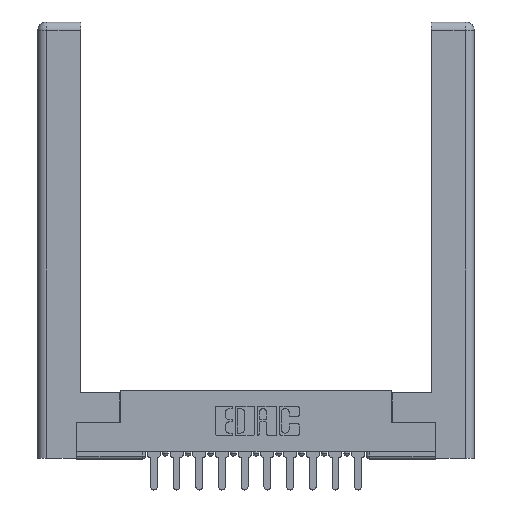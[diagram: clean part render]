
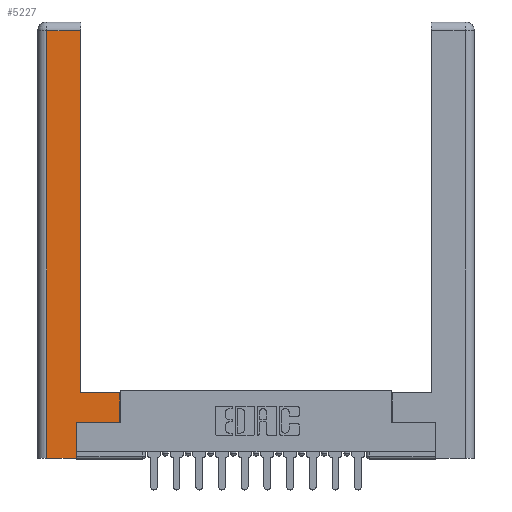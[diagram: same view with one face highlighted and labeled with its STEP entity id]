
A CAD part, top view. The second image highlights one B-rep face of the part: STEP entity #5227.
In plain terms, the highlighted planar face has unit normal (0, 0, 1).
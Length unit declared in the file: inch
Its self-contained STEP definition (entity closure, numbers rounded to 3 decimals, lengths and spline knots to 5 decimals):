
#291 = CARTESIAN_POINT ( 'NONE',  ( 0.0615, 0., 0. ) ) ;
#325 = CARTESIAN_POINT ( 'NONE',  ( 0.265, 0., 0. ) ) ;
#368 = ORIENTED_EDGE ( 'NONE', *, *, #6284, .T. ) ;
#783 = VERTEX_POINT ( 'NONE', #10600 ) ;
#956 = CARTESIAN_POINT ( 'NONE',  ( 0.565, 0.245, 0. ) ) ;
#1530 = VECTOR ( 'NONE', #2260, 39.37008 ) ;
#1540 = VECTOR ( 'NONE', #11471, 39.37008 ) ;
#1660 = ORIENTED_EDGE ( 'NONE', *, *, #10206, .T. ) ;
#2072 = ORIENTED_EDGE ( 'NONE', *, *, #11673, .T. ) ;
#2087 = LINE ( 'NONE', #2231, #9474 ) ;
#2155 = DIRECTION ( 'NONE',  ( -1., 0., 0. ) ) ;
#2202 = DIRECTION ( 'NONE',  ( -1., 0., 0. ) ) ;
#2231 = CARTESIAN_POINT ( 'NONE',  ( 0.295, 3., 0. ) ) ;
#2260 = DIRECTION ( 'NONE',  ( 0., 1., 0. ) ) ;
#2530 = EDGE_CURVE ( 'NONE', #13134, #783, #7236, .T. ) ;
#2780 = LINE ( 'NONE', #5709, #1530 ) ;
#2924 = EDGE_CURVE ( 'NONE', #9411, #13294, #2087, .T. ) ;
#3008 = EDGE_CURVE ( 'NONE', #9317, #10357, #3397, .T. ) ;
#3238 = DIRECTION ( 'NONE',  ( 0., 1., 0. ) ) ;
#3397 = LINE ( 'NONE', #10175, #13503 ) ;
#3718 = CARTESIAN_POINT ( 'NONE',  ( 0.565, 0.45, 0. ) ) ;
#3811 = DIRECTION ( 'NONE',  ( 1., 0., 0. ) ) ;
#3886 = DIRECTION ( 'NONE',  ( 0., 0., -1. ) ) ;
#4324 = DIRECTION ( 'NONE',  ( 0., 1., 0. ) ) ;
#4502 = EDGE_CURVE ( 'NONE', #8087, #12818, #2780, .T. ) ;
#4535 = VECTOR ( 'NONE', #2155, 39.37008 ) ;
#4922 = DIRECTION ( 'NONE',  ( 0., -1., 0. ) ) ;
#5039 = FACE_OUTER_BOUND ( 'NONE', #12690, .T. ) ;
#5227 = ADVANCED_FACE ( 'NONE', ( #5039 ), #9749, .F. ) ;
#5663 = CARTESIAN_POINT ( 'NONE',  ( 0.0615, 2.94, 0. ) ) ;
#5709 = CARTESIAN_POINT ( 'NONE',  ( 0.265, 0.245, 0. ) ) ;
#6284 = EDGE_CURVE ( 'NONE', #12818, #9317, #10082, .T. ) ;
#6409 = CARTESIAN_POINT ( 'NONE',  ( 0.0615, 2.94, 0. ) ) ;
#6525 = ORIENTED_EDGE ( 'NONE', *, *, #2924, .T. ) ;
#6530 = VECTOR ( 'NONE', #4922, 39.37008 ) ;
#6611 = CARTESIAN_POINT ( 'NONE',  ( 0.565, 0.245, 0. ) ) ;
#6668 = AXIS2_PLACEMENT_3D ( 'NONE', #14415, #3886, #8582 ) ;
#7236 = LINE ( 'NONE', #291, #6530 ) ;
#7510 = LINE ( 'NONE', #325, #11706 ) ;
#7615 = ORIENTED_EDGE ( 'NONE', *, *, #4502, .T. ) ;
#7645 = CARTESIAN_POINT ( 'NONE',  ( 0.295, 0.45, 0. ) ) ;
#7831 = CARTESIAN_POINT ( 'NONE',  ( 0.295, 0.45, 0. ) ) ;
#8087 = VERTEX_POINT ( 'NONE', #14678 ) ;
#8182 = ORIENTED_EDGE ( 'NONE', *, *, #13422, .T. ) ;
#8305 = CARTESIAN_POINT ( 'NONE',  ( 0.265, 0.245, 0. ) ) ;
#8582 = DIRECTION ( 'NONE',  ( -1., 0., 0. ) ) ;
#8696 = LINE ( 'NONE', #7831, #9165 ) ;
#9165 = VECTOR ( 'NONE', #2202, 39.37008 ) ;
#9317 = VERTEX_POINT ( 'NONE', #6611 ) ;
#9411 = VERTEX_POINT ( 'NONE', #7645 ) ;
#9474 = VECTOR ( 'NONE', #3238, 39.37008 ) ;
#9580 = CARTESIAN_POINT ( 'NONE',  ( 0.295, 2.94, 0. ) ) ;
#9749 = PLANE ( 'NONE',  #6668 ) ;
#10050 = ORIENTED_EDGE ( 'NONE', *, *, #2530, .T. ) ;
#10082 = LINE ( 'NONE', #956, #1540 ) ;
#10175 = CARTESIAN_POINT ( 'NONE',  ( 0.565, 0.45, 0. ) ) ;
#10206 = EDGE_CURVE ( 'NONE', #10357, #9411, #8696, .T. ) ;
#10357 = VERTEX_POINT ( 'NONE', #3718 ) ;
#10597 = LINE ( 'NONE', #5663, #4535 ) ;
#10600 = CARTESIAN_POINT ( 'NONE',  ( 0.0615, 0., 0. ) ) ;
#11471 = DIRECTION ( 'NONE',  ( 1., 0., 0. ) ) ;
#11673 = EDGE_CURVE ( 'NONE', #13294, #13134, #10597, .T. ) ;
#11706 = VECTOR ( 'NONE', #3811, 39.37008 ) ;
#12690 = EDGE_LOOP ( 'NONE', ( #6525, #2072, #10050, #8182, #7615, #368, #14412, #1660 ) ) ;
#12818 = VERTEX_POINT ( 'NONE', #8305 ) ;
#13134 = VERTEX_POINT ( 'NONE', #6409 ) ;
#13294 = VERTEX_POINT ( 'NONE', #9580 ) ;
#13422 = EDGE_CURVE ( 'NONE', #783, #8087, #7510, .T. ) ;
#13503 = VECTOR ( 'NONE', #4324, 39.37008 ) ;
#14412 = ORIENTED_EDGE ( 'NONE', *, *, #3008, .T. ) ;
#14415 = CARTESIAN_POINT ( 'NONE',  ( 0., 0., 0. ) ) ;
#14678 = CARTESIAN_POINT ( 'NONE',  ( 0.265, 0., 0. ) ) ;
